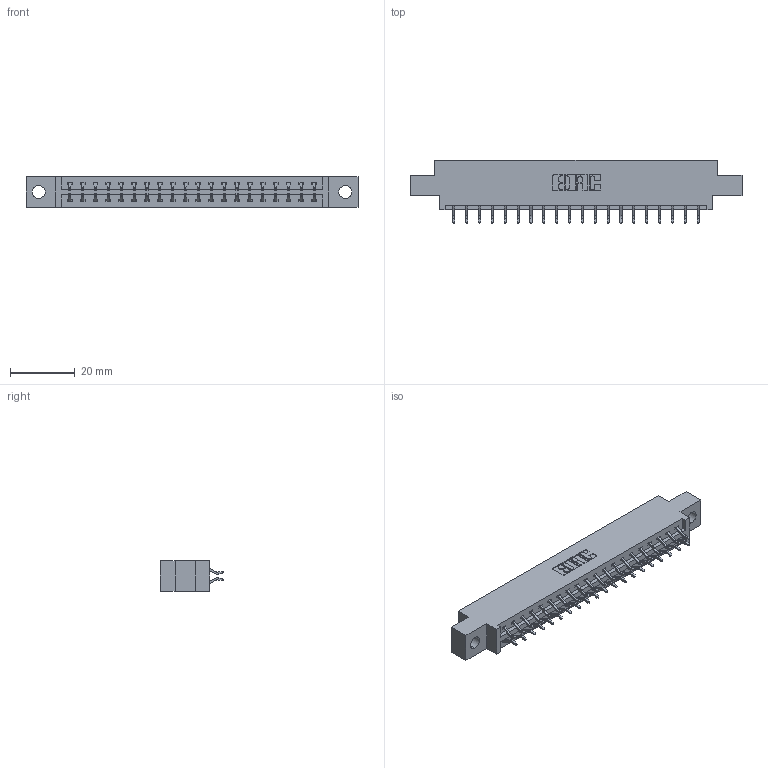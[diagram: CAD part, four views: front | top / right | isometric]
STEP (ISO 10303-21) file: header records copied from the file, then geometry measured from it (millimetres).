
FILE_DESCRIPTION (( 'STEP AP203' ), '1' );
FILE_NAME ('337-040-556-804.STEP', '2019-10-11T12:17:58', ( '' ), ( '' ), 'SwSTEP 2.0', 'SolidWorks 2016', '' );
FILE_SCHEMA (( 'CONFIG_CONTROL_DESIGN' ));
Length unit declared in the file: inch
Products named in the file (3): 337-040-556-804; 337 Part_0.170 Offset - 0.156 Dia-TH; 345-292-001_556 Tail
Assembly tree (41 placements, depth 2):
  337-040-556-804
    337 Part_0.170 Offset - 0.156 Dia-TH
    345-292-001_556 Tail  x40
Bounding box: 102.26 x 19.57 x 9.4 mm (x, y, z)
Volume: 10277.2 mm3; surface area: 11267.7 mm2
Topology: 41 solids, 41 shells, 2518 faces, 7483 edges, 4934 vertices
Faces by surface type: plane 1754, cylinder 764
Entity records: 18707 total; most frequent: CARTESIAN_POINT 3186, ORIENTED_EDGE 3110, DIRECTION 2739, EDGE_CURVE 1555, LINE 1419, VECTOR 1419, VERTEX_POINT 1034, AXIS2_PLACEMENT_3D 660
